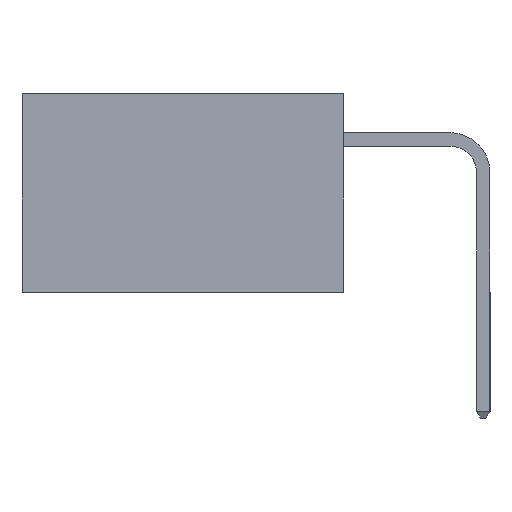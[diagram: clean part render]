
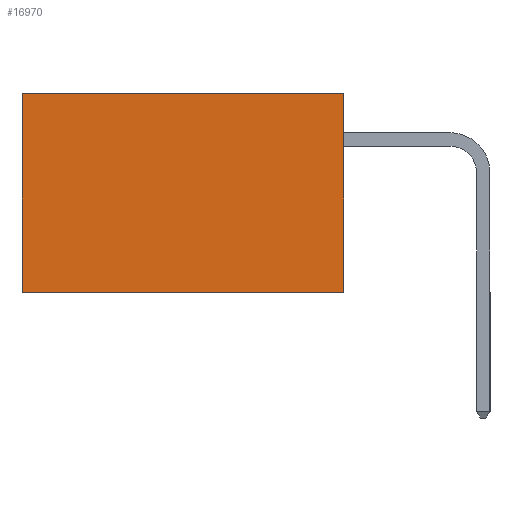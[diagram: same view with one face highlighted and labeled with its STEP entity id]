
A CAD part, left-side view. The second image highlights one B-rep face of the part: STEP entity #16970.
In plain terms, the highlighted planar face has unit normal (-1, 0, 0).
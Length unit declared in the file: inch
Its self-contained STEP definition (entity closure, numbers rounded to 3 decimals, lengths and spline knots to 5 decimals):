
#613 = FACE_OUTER_BOUND ( 'NONE', #27649, .T. ) ;
#2361 = CARTESIAN_POINT ( 'NONE',  ( 0.298, 0.6, 0. ) ) ;
#3453 = DIRECTION ( 'NONE',  ( 0., 0., -1. ) ) ;
#3666 = VECTOR ( 'NONE', #8991, 39.37008 ) ;
#4128 = EDGE_CURVE ( 'NONE', #14397, #23724, #5742, .T. ) ;
#5101 = LINE ( 'NONE', #15570, #16549 ) ;
#5172 = DIRECTION ( 'NONE',  ( 0., 0., -1. ) ) ;
#5742 = LINE ( 'NONE', #28959, #17961 ) ;
#7368 = LINE ( 'NONE', #24555, #19563 ) ;
#8991 = DIRECTION ( 'NONE',  ( 0., 1., 0. ) ) ;
#10800 = CARTESIAN_POINT ( 'NONE',  ( 0.298, 0., 0. ) ) ;
#10863 = EDGE_CURVE ( 'NONE', #30425, #20228, #15863, .T. ) ;
#13345 = DIRECTION ( 'NONE',  ( 0., 0., -1. ) ) ;
#14397 = VERTEX_POINT ( 'NONE', #28725 ) ;
#15203 = AXIS2_PLACEMENT_3D ( 'NONE', #10800, #28003, #13345 ) ;
#15570 = CARTESIAN_POINT ( 'NONE',  ( 0.298, 0.6, 0. ) ) ;
#15863 = LINE ( 'NONE', #23559, #3666 ) ;
#16549 = VECTOR ( 'NONE', #3453, 39.37008 ) ;
#16970 = ADVANCED_FACE ( 'NONE', ( #613 ), #25506, .F. ) ;
#17961 = VECTOR ( 'NONE', #28578, 39.37008 ) ;
#18064 = EDGE_CURVE ( 'NONE', #30425, #14397, #7368, .T. ) ;
#19563 = VECTOR ( 'NONE', #5172, 39.37008 ) ;
#19761 = ORIENTED_EDGE ( 'NONE', *, *, #18064, .F. ) ;
#20228 = VERTEX_POINT ( 'NONE', #2361 ) ;
#21985 = CARTESIAN_POINT ( 'NONE',  ( 0.298, 0.6, -0.37 ) ) ;
#23559 = CARTESIAN_POINT ( 'NONE',  ( 0.298, 0., 0. ) ) ;
#23724 = VERTEX_POINT ( 'NONE', #21985 ) ;
#24445 = ORIENTED_EDGE ( 'NONE', *, *, #29038, .T. ) ;
#24555 = CARTESIAN_POINT ( 'NONE',  ( 0.298, 0., 0. ) ) ;
#25506 = PLANE ( 'NONE',  #15203 ) ;
#27649 = EDGE_LOOP ( 'NONE', ( #24445, #29262, #19761, #28500 ) ) ;
#28003 = DIRECTION ( 'NONE',  ( 1., 0., 0. ) ) ;
#28500 = ORIENTED_EDGE ( 'NONE', *, *, #10863, .T. ) ;
#28578 = DIRECTION ( 'NONE',  ( 0., 1., 0. ) ) ;
#28725 = CARTESIAN_POINT ( 'NONE',  ( 0.298, 0., -0.37 ) ) ;
#28959 = CARTESIAN_POINT ( 'NONE',  ( 0.298, 0., -0.37 ) ) ;
#29038 = EDGE_CURVE ( 'NONE', #20228, #23724, #5101, .T. ) ;
#29262 = ORIENTED_EDGE ( 'NONE', *, *, #4128, .F. ) ;
#30425 = VERTEX_POINT ( 'NONE', #30840 ) ;
#30840 = CARTESIAN_POINT ( 'NONE',  ( 0.298, 0., 0. ) ) ;
